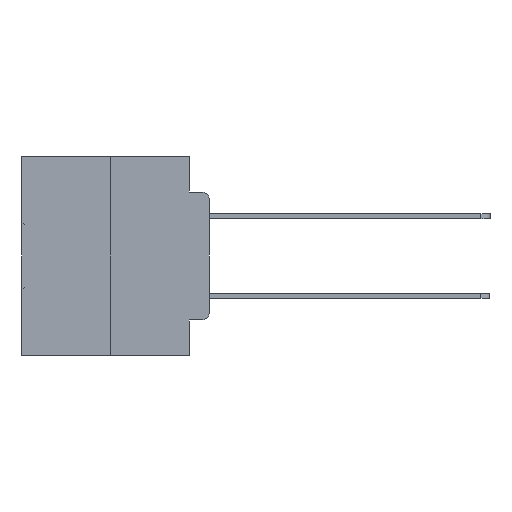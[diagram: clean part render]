
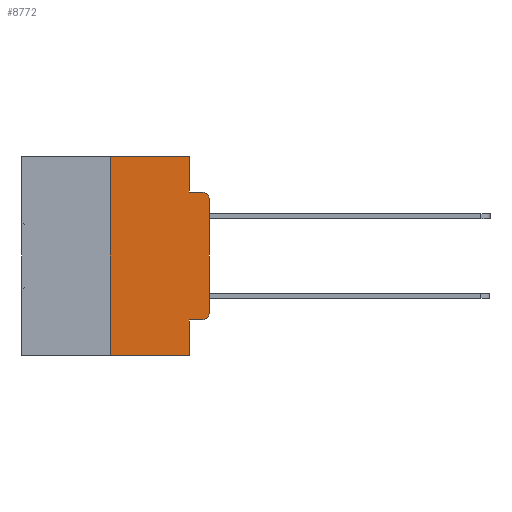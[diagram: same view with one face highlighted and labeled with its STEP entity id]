
A CAD part, left-side view. The second image highlights one B-rep face of the part: STEP entity #8772.
In plain terms, the highlighted planar face has unit normal (-1, 0, 0).
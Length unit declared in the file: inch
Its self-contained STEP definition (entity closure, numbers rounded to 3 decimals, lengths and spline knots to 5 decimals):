
#73 = CARTESIAN_POINT ( 'NONE',  ( 0., 0., 0. ) ) ;
#542 = DIRECTION ( 'NONE',  ( 0., 0., -1. ) ) ;
#1075 = CARTESIAN_POINT ( 'NONE',  ( 0., 0.02, -0.3915 ) ) ;
#1144 = CARTESIAN_POINT ( 'NONE',  ( 0., 0.051, 0. ) ) ;
#1228 = ORIENTED_EDGE ( 'NONE', *, *, #21224, .T. ) ;
#1816 = CARTESIAN_POINT ( 'NONE',  ( 0., 0.051, -0.0885 ) ) ;
#2136 = EDGE_CURVE ( 'NONE', #10294, #8615, #24789, .T. ) ;
#2406 = CARTESIAN_POINT ( 'NONE',  ( 0., 0.473, -0.5 ) ) ;
#3753 = DIRECTION ( 'NONE',  ( 0., 0., -1. ) ) ;
#3813 = DIRECTION ( 'NONE',  ( 0., 0., -1. ) ) ;
#3831 = VERTEX_POINT ( 'NONE', #6549 ) ;
#4275 = VERTEX_POINT ( 'NONE', #1816 ) ;
#4359 = CARTESIAN_POINT ( 'NONE',  ( 0., 0.051, -0.4115 ) ) ;
#4800 = EDGE_CURVE ( 'NONE', #4275, #21935, #28630, .T. ) ;
#4974 = CARTESIAN_POINT ( 'NONE',  ( 0., 0., -0.3915 ) ) ;
#6116 = VERTEX_POINT ( 'NONE', #25014 ) ;
#6155 = CARTESIAN_POINT ( 'NONE',  ( 0., 0.051, 0. ) ) ;
#6236 = CARTESIAN_POINT ( 'NONE',  ( 0., 0.02, -0.4115 ) ) ;
#6253 = LINE ( 'NONE', #25954, #26041 ) ;
#6549 = CARTESIAN_POINT ( 'NONE',  ( 0., 0.25, 0. ) ) ;
#6608 = PLANE ( 'NONE',  #21397 ) ;
#6792 = CARTESIAN_POINT ( 'NONE',  ( 0., 0.051, -0.0885 ) ) ;
#6823 = CARTESIAN_POINT ( 'NONE',  ( 0., 0.473, 0. ) ) ;
#7362 = DIRECTION ( 'NONE',  ( -1., 0., 0. ) ) ;
#7446 = CARTESIAN_POINT ( 'NONE',  ( 0., 0.25, -0.5 ) ) ;
#7571 = VECTOR ( 'NONE', #20281, 39.37008 ) ;
#8615 = VERTEX_POINT ( 'NONE', #11022 ) ;
#8772 = ADVANCED_FACE ( 'NONE', ( #20956 ), #6608, .F. ) ;
#9094 = LINE ( 'NONE', #21399, #15900 ) ;
#9310 = VERTEX_POINT ( 'NONE', #6236 ) ;
#9438 = DIRECTION ( 'NONE',  ( 0., -1., 0. ) ) ;
#10291 = ORIENTED_EDGE ( 'NONE', *, *, #19503, .F. ) ;
#10294 = VERTEX_POINT ( 'NONE', #4974 ) ;
#10430 = CARTESIAN_POINT ( 'NONE',  ( 0., 0.051, -0.4115 ) ) ;
#11022 = CARTESIAN_POINT ( 'NONE',  ( 0., 0., -0.1085 ) ) ;
#11786 = DIRECTION ( 'NONE',  ( 1., 0., 0. ) ) ;
#11915 = EDGE_CURVE ( 'NONE', #22301, #4275, #9094, .T. ) ;
#12788 = DIRECTION ( 'NONE',  ( 0., -1., 0. ) ) ;
#13023 = LINE ( 'NONE', #1144, #19123 ) ;
#13514 = ORIENTED_EDGE ( 'NONE', *, *, #32332, .T. ) ;
#14577 = CIRCLE ( 'NONE', #19736, 0.02 ) ;
#15900 = VECTOR ( 'NONE', #542, 39.37008 ) ;
#17039 = LINE ( 'NONE', #2406, #30701 ) ;
#17548 = CIRCLE ( 'NONE', #24389, 0.02 ) ;
#17917 = VECTOR ( 'NONE', #25429, 39.37008 ) ;
#17957 = ORIENTED_EDGE ( 'NONE', *, *, #20649, .T. ) ;
#18350 = EDGE_CURVE ( 'NONE', #3831, #22301, #31627, .T. ) ;
#19123 = VECTOR ( 'NONE', #3813, 39.37008 ) ;
#19327 = DIRECTION ( 'NONE',  ( -1., 0., 0. ) ) ;
#19487 = CARTESIAN_POINT ( 'NONE',  ( 0., 0.473, 0. ) ) ;
#19503 = EDGE_CURVE ( 'NONE', #31695, #3831, #6253, .T. ) ;
#19736 = AXIS2_PLACEMENT_3D ( 'NONE', #22821, #7362, #25404 ) ;
#20281 = DIRECTION ( 'NONE',  ( 0., -1., 0. ) ) ;
#20353 = EDGE_CURVE ( 'NONE', #26359, #6116, #13023, .T. ) ;
#20649 = EDGE_CURVE ( 'NONE', #31695, #6116, #17039, .T. ) ;
#20746 = CARTESIAN_POINT ( 'NONE',  ( 0., 0.02, -0.0885 ) ) ;
#20956 = FACE_OUTER_BOUND ( 'NONE', #22335, .T. ) ;
#21224 = EDGE_CURVE ( 'NONE', #8615, #21935, #14577, .T. ) ;
#21397 = AXIS2_PLACEMENT_3D ( 'NONE', #19487, #11786, #29785 ) ;
#21399 = CARTESIAN_POINT ( 'NONE',  ( 0., 0.051, 0. ) ) ;
#21935 = VERTEX_POINT ( 'NONE', #20746 ) ;
#22020 = ORIENTED_EDGE ( 'NONE', *, *, #28957, .T. ) ;
#22095 = LINE ( 'NONE', #10430, #7571 ) ;
#22301 = VERTEX_POINT ( 'NONE', #6155 ) ;
#22335 = EDGE_LOOP ( 'NONE', ( #30770, #1228, #32779, #26853, #28448, #10291, #17957, #26462, #13514, #22020 ) ) ;
#22821 = CARTESIAN_POINT ( 'NONE',  ( 0., 0.02, -0.1085 ) ) ;
#24057 = VECTOR ( 'NONE', #9438, 39.37008 ) ;
#24389 = AXIS2_PLACEMENT_3D ( 'NONE', #1075, #19327, #3753 ) ;
#24789 = LINE ( 'NONE', #73, #17917 ) ;
#24847 = DIRECTION ( 'NONE',  ( 0., -1., 0. ) ) ;
#25014 = CARTESIAN_POINT ( 'NONE',  ( 0., 0.051, -0.5 ) ) ;
#25404 = DIRECTION ( 'NONE',  ( 0., 0., -1. ) ) ;
#25429 = DIRECTION ( 'NONE',  ( 0., 0., 1. ) ) ;
#25954 = CARTESIAN_POINT ( 'NONE',  ( 0., 0.25, 0. ) ) ;
#26041 = VECTOR ( 'NONE', #28525, 39.37008 ) ;
#26359 = VERTEX_POINT ( 'NONE', #4359 ) ;
#26462 = ORIENTED_EDGE ( 'NONE', *, *, #20353, .F. ) ;
#26853 = ORIENTED_EDGE ( 'NONE', *, *, #11915, .F. ) ;
#28448 = ORIENTED_EDGE ( 'NONE', *, *, #18350, .F. ) ;
#28525 = DIRECTION ( 'NONE',  ( 0., 0., 1. ) ) ;
#28630 = LINE ( 'NONE', #6792, #30985 ) ;
#28957 = EDGE_CURVE ( 'NONE', #9310, #10294, #17548, .T. ) ;
#29785 = DIRECTION ( 'NONE',  ( 0., 0., -1. ) ) ;
#30701 = VECTOR ( 'NONE', #12788, 39.37008 ) ;
#30770 = ORIENTED_EDGE ( 'NONE', *, *, #2136, .T. ) ;
#30985 = VECTOR ( 'NONE', #24847, 39.37008 ) ;
#31627 = LINE ( 'NONE', #6823, #24057 ) ;
#31695 = VERTEX_POINT ( 'NONE', #7446 ) ;
#32332 = EDGE_CURVE ( 'NONE', #26359, #9310, #22095, .T. ) ;
#32779 = ORIENTED_EDGE ( 'NONE', *, *, #4800, .F. ) ;
